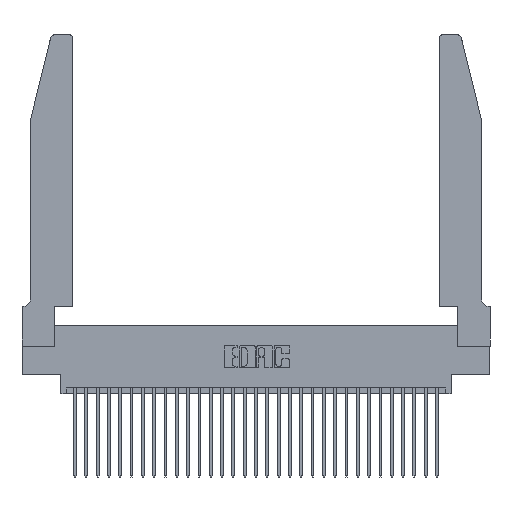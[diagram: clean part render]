
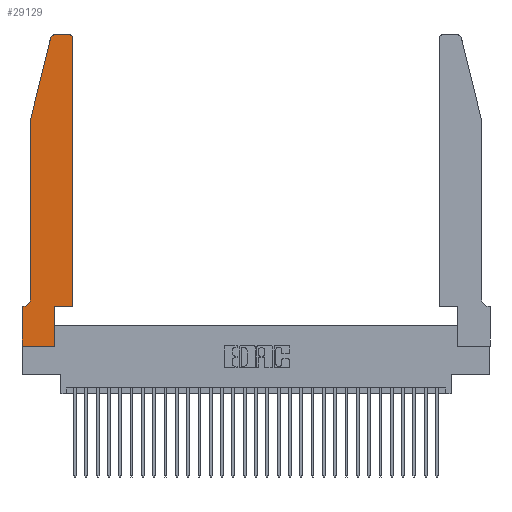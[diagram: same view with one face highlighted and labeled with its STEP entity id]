
A CAD part, top view. The second image highlights one B-rep face of the part: STEP entity #29129.
In plain terms, the highlighted planar face has unit normal (0, 0, 1).
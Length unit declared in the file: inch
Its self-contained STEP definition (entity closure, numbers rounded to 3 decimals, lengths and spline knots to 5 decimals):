
#334 = VERTEX_POINT ( 'NONE', #26236 ) ;
#744 = LINE ( 'NONE', #7534, #20622 ) ;
#1115 = EDGE_CURVE ( 'NONE', #4571, #27497, #2059, .T. ) ;
#1518 = DIRECTION ( 'NONE',  ( 1., 0., 0. ) ) ;
#1988 = VECTOR ( 'NONE', #16746, 39.37008 ) ;
#2059 = CIRCLE ( 'NONE', #31218, 0.03 ) ;
#2887 = EDGE_CURVE ( 'NONE', #27974, #14957, #744, .T. ) ;
#3733 = CARTESIAN_POINT ( 'NONE',  ( 0.4505, 2.72, 0.37 ) ) ;
#3892 = EDGE_CURVE ( 'NONE', #16901, #334, #5834, .T. ) ;
#4571 = VERTEX_POINT ( 'NONE', #19047 ) ;
#4679 = VECTOR ( 'NONE', #10944, 39.37008 ) ;
#4856 = VERTEX_POINT ( 'NONE', #28571 ) ;
#4969 = CIRCLE ( 'NONE', #10667, 0.03 ) ;
#5115 = ORIENTED_EDGE ( 'NONE', *, *, #3892, .T. ) ;
#5155 = CARTESIAN_POINT ( 'NONE',  ( 0.4205, 2.72, 0.37 ) ) ;
#5285 = LINE ( 'NONE', #20670, #24218 ) ;
#5690 = CARTESIAN_POINT ( 'NONE',  ( 0.4505, 0.35, 0.37 ) ) ;
#5822 = LINE ( 'NONE', #5690, #31224 ) ;
#5833 = CARTESIAN_POINT ( 'NONE',  ( 0.2865, 0., 0.37 ) ) ;
#5834 = LINE ( 'NONE', #21423, #18286 ) ;
#6014 = LINE ( 'NONE', #25351, #19215 ) ;
#6708 = DIRECTION ( 'NONE',  ( 0., 0., 1. ) ) ;
#7044 = ORIENTED_EDGE ( 'NONE', *, *, #2887, .T. ) ;
#7369 = CARTESIAN_POINT ( 'NONE',  ( 0.0755, 2., 0.37 ) ) ;
#7534 = CARTESIAN_POINT ( 'NONE',  ( 0., 0., 0.37 ) ) ;
#7562 = ORIENTED_EDGE ( 'NONE', *, *, #23046, .T. ) ;
#7692 = DIRECTION ( 'NONE',  ( 1., 0., 0. ) ) ;
#8146 = ORIENTED_EDGE ( 'NONE', *, *, #15234, .T. ) ;
#8577 = ORIENTED_EDGE ( 'NONE', *, *, #9410, .T. ) ;
#9093 = CARTESIAN_POINT ( 'NONE',  ( 0.0055, 0.42, 0.37 ) ) ;
#9398 = CARTESIAN_POINT ( 'NONE',  ( 0., 0., 0.37 ) ) ;
#9410 = EDGE_CURVE ( 'NONE', #14957, #16901, #5285, .T. ) ;
#9542 = VERTEX_POINT ( 'NONE', #3733 ) ;
#9627 = VERTEX_POINT ( 'NONE', #16548 ) ;
#10015 = CARTESIAN_POINT ( 'NONE',  ( 0.0755, 2., 0.37 ) ) ;
#10189 = ORIENTED_EDGE ( 'NONE', *, *, #10272, .T. ) ;
#10272 = EDGE_CURVE ( 'NONE', #12088, #18810, #25682, .T. ) ;
#10654 = DIRECTION ( 'NONE',  ( 0., -1., 0. ) ) ;
#10667 = AXIS2_PLACEMENT_3D ( 'NONE', #5155, #22471, #7692 ) ;
#10944 = DIRECTION ( 'NONE',  ( -1., 0., 0. ) ) ;
#11427 = CARTESIAN_POINT ( 'NONE',  ( 0.0055, 0.35, 0.37 ) ) ;
#11594 = DIRECTION ( 'NONE',  ( -1., 0., 0. ) ) ;
#12088 = VERTEX_POINT ( 'NONE', #15489 ) ;
#12524 = ORIENTED_EDGE ( 'NONE', *, *, #31448, .T. ) ;
#14201 = AXIS2_PLACEMENT_3D ( 'NONE', #9093, #26286, #11594 ) ;
#14957 = VERTEX_POINT ( 'NONE', #5833 ) ;
#15234 = EDGE_CURVE ( 'NONE', #4856, #4571, #21820, .T. ) ;
#15489 = CARTESIAN_POINT ( 'NONE',  ( 0.0755, 0.42, 0.37 ) ) ;
#16548 = CARTESIAN_POINT ( 'NONE',  ( 0., 0.35, 0.37 ) ) ;
#16650 = PLANE ( 'NONE',  #23193 ) ;
#16746 = DIRECTION ( 'NONE',  ( -1., 0., 0. ) ) ;
#16901 = VERTEX_POINT ( 'NONE', #23354 ) ;
#16940 = ORIENTED_EDGE ( 'NONE', *, *, #23003, .T. ) ;
#18136 = DIRECTION ( 'NONE',  ( 0., 1., 0. ) ) ;
#18179 = LINE ( 'NONE', #19077, #30366 ) ;
#18286 = VECTOR ( 'NONE', #1518, 39.37008 ) ;
#18810 = VERTEX_POINT ( 'NONE', #11427 ) ;
#19047 = CARTESIAN_POINT ( 'NONE',  ( 0.284, 2.75, 0.37 ) ) ;
#19077 = CARTESIAN_POINT ( 'NONE',  ( 0., 0., 0.37 ) ) ;
#19172 = VERTEX_POINT ( 'NONE', #10015 ) ;
#19215 = VECTOR ( 'NONE', #10654, 39.37008 ) ;
#19303 = CARTESIAN_POINT ( 'NONE',  ( 0.284, 2.72, 0.37 ) ) ;
#20521 = DIRECTION ( 'NONE',  ( 0., 1., 0. ) ) ;
#20619 = DIRECTION ( 'NONE',  ( 0., 0., 1. ) ) ;
#20622 = VECTOR ( 'NONE', #24768, 39.37008 ) ;
#20670 = CARTESIAN_POINT ( 'NONE',  ( 0.2865, 0.35, 0.37 ) ) ;
#21423 = CARTESIAN_POINT ( 'NONE',  ( 0.4505, 0.35, 0.37 ) ) ;
#21522 = CARTESIAN_POINT ( 'NONE',  ( 0., 0.35, 0.37 ) ) ;
#21820 = LINE ( 'NONE', #26417, #1988 ) ;
#22066 = EDGE_CURVE ( 'NONE', #334, #9542, #5822, .T. ) ;
#22471 = DIRECTION ( 'NONE',  ( 0., 0., 1. ) ) ;
#23003 = EDGE_CURVE ( 'NONE', #27497, #19172, #31928, .T. ) ;
#23046 = EDGE_CURVE ( 'NONE', #9542, #4856, #4969, .T. ) ;
#23184 = ORIENTED_EDGE ( 'NONE', *, *, #27130, .T. ) ;
#23193 = AXIS2_PLACEMENT_3D ( 'NONE', #21522, #6708, #23967 ) ;
#23354 = CARTESIAN_POINT ( 'NONE',  ( 0.2865, 0.35, 0.37 ) ) ;
#23756 = ORIENTED_EDGE ( 'NONE', *, *, #29145, .T. ) ;
#23967 = DIRECTION ( 'NONE',  ( 1., 0., 0. ) ) ;
#24218 = VECTOR ( 'NONE', #18136, 39.37008 ) ;
#24768 = DIRECTION ( 'NONE',  ( 1., 0., 0. ) ) ;
#25351 = CARTESIAN_POINT ( 'NONE',  ( 0.0755, 2., 0.37 ) ) ;
#25682 = CIRCLE ( 'NONE', #14201, 0.07 ) ;
#26217 = VECTOR ( 'NONE', #27186, 39.37008 ) ;
#26236 = CARTESIAN_POINT ( 'NONE',  ( 0.4505, 0.35, 0.37 ) ) ;
#26286 = DIRECTION ( 'NONE',  ( 0., 0., -1. ) ) ;
#26417 = CARTESIAN_POINT ( 'NONE',  ( 0.2605, 2.75, 0.37 ) ) ;
#26838 = ORIENTED_EDGE ( 'NONE', *, *, #22066, .T. ) ;
#27130 = EDGE_CURVE ( 'NONE', #18810, #9627, #30878, .T. ) ;
#27186 = DIRECTION ( 'NONE',  ( -0.239, -0.971, 0. ) ) ;
#27248 = CARTESIAN_POINT ( 'NONE',  ( 0.25487, 2.72718, 0.37 ) ) ;
#27497 = VERTEX_POINT ( 'NONE', #27248 ) ;
#27974 = VERTEX_POINT ( 'NONE', #9398 ) ;
#28126 = DIRECTION ( 'NONE',  ( 1., 0., 0. ) ) ;
#28438 = ORIENTED_EDGE ( 'NONE', *, *, #1115, .T. ) ;
#28571 = CARTESIAN_POINT ( 'NONE',  ( 0.4205, 2.75, 0.37 ) ) ;
#29129 = ADVANCED_FACE ( 'NONE', ( #31125 ), #16650, .T. ) ;
#29145 = EDGE_CURVE ( 'NONE', #9627, #27974, #18179, .T. ) ;
#29902 = EDGE_LOOP ( 'NONE', ( #8146, #28438, #16940, #12524, #10189, #23184, #23756, #7044, #8577, #5115, #26838, #7562 ) ) ;
#30366 = VECTOR ( 'NONE', #31320, 39.37008 ) ;
#30538 = CARTESIAN_POINT ( 'NONE',  ( 0.0755, 0.35, 0.37 ) ) ;
#30878 = LINE ( 'NONE', #30538, #4679 ) ;
#31125 = FACE_OUTER_BOUND ( 'NONE', #29902, .T. ) ;
#31218 = AXIS2_PLACEMENT_3D ( 'NONE', #19303, #20619, #28126 ) ;
#31224 = VECTOR ( 'NONE', #20521, 39.37008 ) ;
#31320 = DIRECTION ( 'NONE',  ( 0., -1., 0. ) ) ;
#31448 = EDGE_CURVE ( 'NONE', #19172, #12088, #6014, .T. ) ;
#31928 = LINE ( 'NONE', #7369, #26217 ) ;
